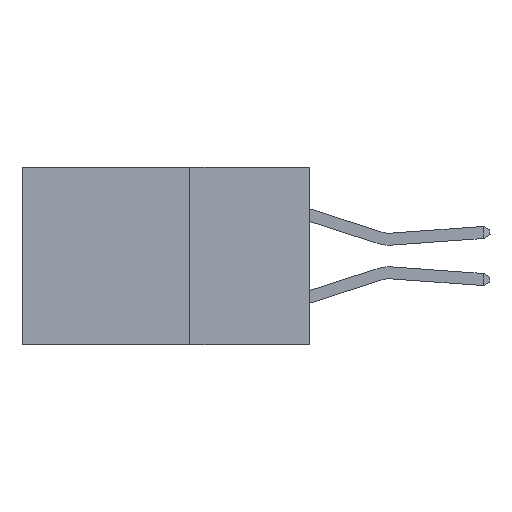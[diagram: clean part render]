
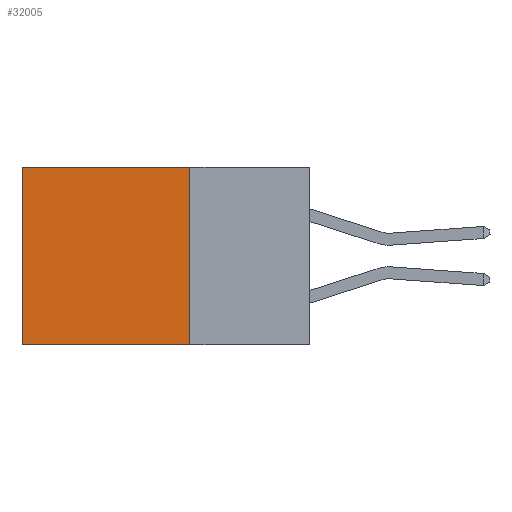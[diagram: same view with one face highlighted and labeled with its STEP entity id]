
A CAD part, left-side view. The second image highlights one B-rep face of the part: STEP entity #32005.
In plain terms, the highlighted planar face has unit normal (-1, 0, 0).
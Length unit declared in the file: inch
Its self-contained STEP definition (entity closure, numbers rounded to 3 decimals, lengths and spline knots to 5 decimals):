
#55 = ORIENTED_EDGE ( 'NONE', *, *, #29032, .F. ) ;
#398 = DIRECTION ( 'NONE',  ( 0., 1., 0. ) ) ;
#701 = EDGE_CURVE ( 'NONE', #17155, #30063, #28801, .T. ) ;
#796 = CARTESIAN_POINT ( 'NONE',  ( 0.298, 0.25, 0. ) ) ;
#1147 = PLANE ( 'NONE',  #15599 ) ;
#1885 = LINE ( 'NONE', #28879, #28060 ) ;
#2144 = ORIENTED_EDGE ( 'NONE', *, *, #13898, .F. ) ;
#4730 = LINE ( 'NONE', #24615, #5529 ) ;
#5529 = VECTOR ( 'NONE', #9332, 39.37008 ) ;
#7116 = CARTESIAN_POINT ( 'NONE',  ( 0.298, 0.6, -0.37 ) ) ;
#8740 = DIRECTION ( 'NONE',  ( 1., 0., 0. ) ) ;
#9332 = DIRECTION ( 'NONE',  ( 0., 1., 0. ) ) ;
#9783 = EDGE_LOOP ( 'NONE', ( #13756, #55, #2144, #10432 ) ) ;
#9850 = CARTESIAN_POINT ( 'NONE',  ( 0.298, 0.6, 0. ) ) ;
#10432 = ORIENTED_EDGE ( 'NONE', *, *, #701, .T. ) ;
#13756 = ORIENTED_EDGE ( 'NONE', *, *, #25446, .T. ) ;
#13898 = EDGE_CURVE ( 'NONE', #17155, #21079, #1885, .T. ) ;
#14931 = LINE ( 'NONE', #9850, #20898 ) ;
#15599 = AXIS2_PLACEMENT_3D ( 'NONE', #24026, #8740, #26565 ) ;
#16530 = FACE_OUTER_BOUND ( 'NONE', #9783, .T. ) ;
#17155 = VERTEX_POINT ( 'NONE', #796 ) ;
#20898 = VECTOR ( 'NONE', #32494, 39.37008 ) ;
#21079 = VERTEX_POINT ( 'NONE', #29249 ) ;
#22088 = VECTOR ( 'NONE', #398, 39.37008 ) ;
#24026 = CARTESIAN_POINT ( 'NONE',  ( 0.298, 0.25, 0. ) ) ;
#24615 = CARTESIAN_POINT ( 'NONE',  ( 0.298, 0.25, -0.37 ) ) ;
#25446 = EDGE_CURVE ( 'NONE', #30063, #26684, #14931, .T. ) ;
#26565 = DIRECTION ( 'NONE',  ( 0., 0., -1. ) ) ;
#26684 = VERTEX_POINT ( 'NONE', #7116 ) ;
#28060 = VECTOR ( 'NONE', #31374, 39.37008 ) ;
#28801 = LINE ( 'NONE', #32063, #22088 ) ;
#28879 = CARTESIAN_POINT ( 'NONE',  ( 0.298, 0.25, 0. ) ) ;
#29032 = EDGE_CURVE ( 'NONE', #21079, #26684, #4730, .T. ) ;
#29249 = CARTESIAN_POINT ( 'NONE',  ( 0.298, 0.25, -0.37 ) ) ;
#30063 = VERTEX_POINT ( 'NONE', #31517 ) ;
#31374 = DIRECTION ( 'NONE',  ( 0., 0., -1. ) ) ;
#31517 = CARTESIAN_POINT ( 'NONE',  ( 0.298, 0.6, 0. ) ) ;
#32005 = ADVANCED_FACE ( 'NONE', ( #16530 ), #1147, .F. ) ;
#32063 = CARTESIAN_POINT ( 'NONE',  ( 0.298, 0.25, 0. ) ) ;
#32494 = DIRECTION ( 'NONE',  ( 0., 0., -1. ) ) ;
